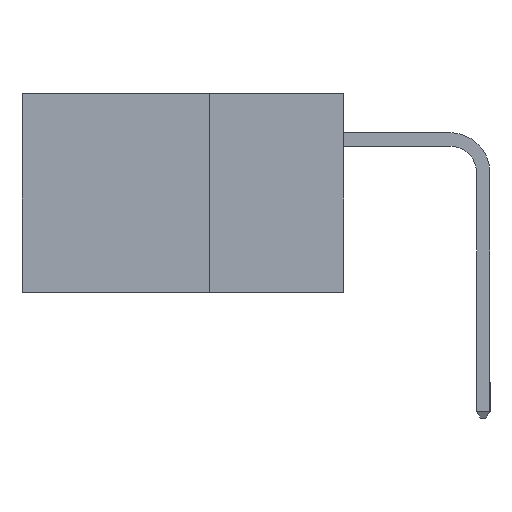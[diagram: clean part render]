
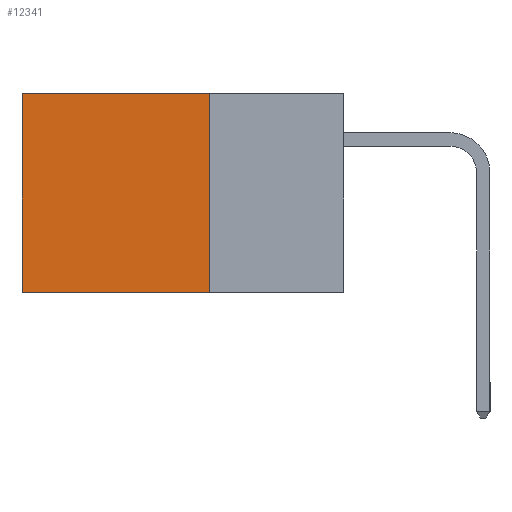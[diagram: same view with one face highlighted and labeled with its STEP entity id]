
A CAD part, left-side view. The second image highlights one B-rep face of the part: STEP entity #12341.
In plain terms, the highlighted planar face has unit normal (-1, 0, 0).
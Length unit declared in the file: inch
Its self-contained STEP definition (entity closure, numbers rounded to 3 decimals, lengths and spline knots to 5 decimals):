
#10 = EDGE_CURVE ( 'NONE', #3991, #13951, #5025, .T. ) ;
#564 = CARTESIAN_POINT ( 'NONE',  ( 0.298, 0.25, 0. ) ) ;
#1291 = AXIS2_PLACEMENT_3D ( 'NONE', #12176, #4522, #13462 ) ;
#1693 = DIRECTION ( 'NONE',  ( 0., 1., 0. ) ) ;
#2190 = DIRECTION ( 'NONE',  ( 0., 0., -1. ) ) ;
#2454 = CARTESIAN_POINT ( 'NONE',  ( 0.298, 0.6, 0. ) ) ;
#2634 = EDGE_LOOP ( 'NONE', ( #6271, #9498, #4799, #5226 ) ) ;
#3223 = PLANE ( 'NONE',  #1291 ) ;
#3980 = DIRECTION ( 'NONE',  ( 0., 0., -1. ) ) ;
#3991 = VERTEX_POINT ( 'NONE', #7752 ) ;
#4522 = DIRECTION ( 'NONE',  ( 1., 0., 0. ) ) ;
#4799 = ORIENTED_EDGE ( 'NONE', *, *, #10, .F. ) ;
#5025 = LINE ( 'NONE', #564, #8461 ) ;
#5226 = ORIENTED_EDGE ( 'NONE', *, *, #6662, .T. ) ;
#5786 = VECTOR ( 'NONE', #2190, 39.37008 ) ;
#6271 = ORIENTED_EDGE ( 'NONE', *, *, #7600, .T. ) ;
#6662 = EDGE_CURVE ( 'NONE', #3991, #7269, #10456, .T. ) ;
#6770 = LINE ( 'NONE', #12320, #9841 ) ;
#7269 = VERTEX_POINT ( 'NONE', #16087 ) ;
#7417 = VECTOR ( 'NONE', #1693, 39.37008 ) ;
#7600 = EDGE_CURVE ( 'NONE', #7269, #13016, #15820, .T. ) ;
#7752 = CARTESIAN_POINT ( 'NONE',  ( 0.298, 0.25, 0. ) ) ;
#8461 = VECTOR ( 'NONE', #3980, 39.37008 ) ;
#9498 = ORIENTED_EDGE ( 'NONE', *, *, #12423, .F. ) ;
#9841 = VECTOR ( 'NONE', #13633, 39.37008 ) ;
#10456 = LINE ( 'NONE', #10979, #7417 ) ;
#10979 = CARTESIAN_POINT ( 'NONE',  ( 0.298, 0.25, 0. ) ) ;
#11029 = CARTESIAN_POINT ( 'NONE',  ( 0.298, 0.25, -0.37 ) ) ;
#11397 = FACE_OUTER_BOUND ( 'NONE', #2634, .T. ) ;
#12176 = CARTESIAN_POINT ( 'NONE',  ( 0.298, 0.25, 0. ) ) ;
#12207 = CARTESIAN_POINT ( 'NONE',  ( 0.298, 0.6, -0.37 ) ) ;
#12320 = CARTESIAN_POINT ( 'NONE',  ( 0.298, 0.25, -0.37 ) ) ;
#12341 = ADVANCED_FACE ( 'NONE', ( #11397 ), #3223, .F. ) ;
#12423 = EDGE_CURVE ( 'NONE', #13951, #13016, #6770, .T. ) ;
#13016 = VERTEX_POINT ( 'NONE', #12207 ) ;
#13462 = DIRECTION ( 'NONE',  ( 0., 0., -1. ) ) ;
#13633 = DIRECTION ( 'NONE',  ( 0., 1., 0. ) ) ;
#13951 = VERTEX_POINT ( 'NONE', #11029 ) ;
#15820 = LINE ( 'NONE', #2454, #5786 ) ;
#16087 = CARTESIAN_POINT ( 'NONE',  ( 0.298, 0.6, 0. ) ) ;
